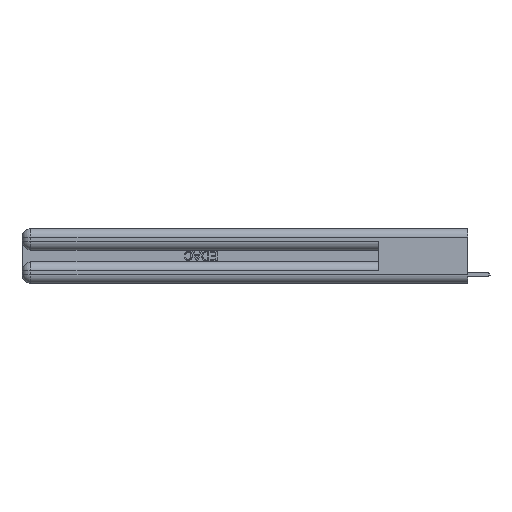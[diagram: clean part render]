
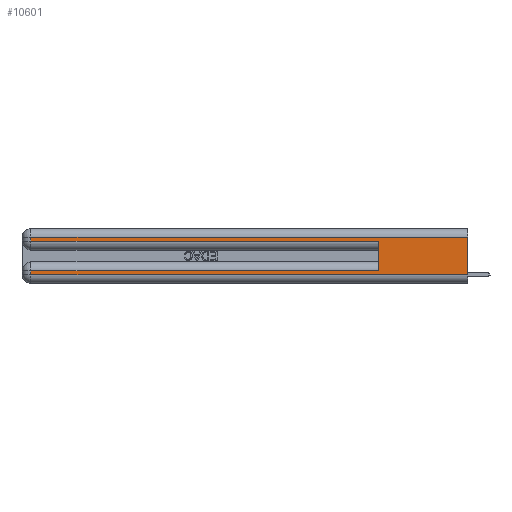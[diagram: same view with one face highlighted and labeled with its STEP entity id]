
A CAD part, left-side view. The second image highlights one B-rep face of the part: STEP entity #10601.
In plain terms, the highlighted planar face has unit normal (-1, 0, 0).
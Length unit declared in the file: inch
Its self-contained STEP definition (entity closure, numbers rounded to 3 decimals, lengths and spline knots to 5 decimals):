
#235 = DIRECTION ( 'NONE',  ( 0., 1., 0. ) ) ;
#849 = VECTOR ( 'NONE', #20794, 39.37008 ) ;
#1959 = VERTEX_POINT ( 'NONE', #27215 ) ;
#2513 = EDGE_CURVE ( 'NONE', #26763, #18658, #7980, .T. ) ;
#3380 = VECTOR ( 'NONE', #11363, 39.37008 ) ;
#3614 = EDGE_CURVE ( 'NONE', #14412, #7182, #16532, .T. ) ;
#3829 = VECTOR ( 'NONE', #19121, 39.37008 ) ;
#3980 = ORIENTED_EDGE ( 'NONE', *, *, #24137, .T. ) ;
#6697 = CARTESIAN_POINT ( 'NONE',  ( 0., 2.94, 0.285 ) ) ;
#7182 = VERTEX_POINT ( 'NONE', #12680 ) ;
#7229 = LINE ( 'NONE', #23382, #849 ) ;
#7321 = CARTESIAN_POINT ( 'NONE',  ( 0., 2.94, 0.37 ) ) ;
#7705 = LINE ( 'NONE', #12514, #15651 ) ;
#7980 = LINE ( 'NONE', #19742, #14417 ) ;
#8640 = ORIENTED_EDGE ( 'NONE', *, *, #27903, .F. ) ;
#8691 = CARTESIAN_POINT ( 'NONE',  ( 0., 0., 0.31 ) ) ;
#8824 = ORIENTED_EDGE ( 'NONE', *, *, #9949, .T. ) ;
#9354 = CARTESIAN_POINT ( 'NONE',  ( 0., 0.6, 0.285 ) ) ;
#9949 = EDGE_CURVE ( 'NONE', #25643, #26763, #21211, .T. ) ;
#9965 = CARTESIAN_POINT ( 'NONE',  ( 0., 2.94, 0.085 ) ) ;
#10220 = CARTESIAN_POINT ( 'NONE',  ( 0., 0., 0.37 ) ) ;
#10309 = LINE ( 'NONE', #19507, #29468 ) ;
#10521 = DIRECTION ( 'NONE',  ( 0., -1., 0. ) ) ;
#10601 = ADVANCED_FACE ( 'NONE', ( #22336 ), #28748, .F. ) ;
#11363 = DIRECTION ( 'NONE',  ( 0., 0., -1. ) ) ;
#12514 = CARTESIAN_POINT ( 'NONE',  ( 0., 0.6, 0.145 ) ) ;
#12680 = CARTESIAN_POINT ( 'NONE',  ( 0., 0., 0.06 ) ) ;
#13570 = VERTEX_POINT ( 'NONE', #9965 ) ;
#14412 = VERTEX_POINT ( 'NONE', #8691 ) ;
#14417 = VECTOR ( 'NONE', #10521, 39.37008 ) ;
#15651 = VECTOR ( 'NONE', #28736, 39.37008 ) ;
#16106 = ORIENTED_EDGE ( 'NONE', *, *, #22147, .T. ) ;
#16199 = EDGE_CURVE ( 'NONE', #13570, #22298, #7229, .T. ) ;
#16532 = LINE ( 'NONE', #10220, #3829 ) ;
#17022 = LINE ( 'NONE', #21890, #26573 ) ;
#17499 = EDGE_CURVE ( 'NONE', #14412, #25643, #27818, .T. ) ;
#17925 = ORIENTED_EDGE ( 'NONE', *, *, #17499, .T. ) ;
#18658 = VERTEX_POINT ( 'NONE', #9354 ) ;
#19046 = ORIENTED_EDGE ( 'NONE', *, *, #16199, .T. ) ;
#19121 = DIRECTION ( 'NONE',  ( 0., 0., -1. ) ) ;
#19507 = CARTESIAN_POINT ( 'NONE',  ( 0., 0., 0.085 ) ) ;
#19614 = DIRECTION ( 'NONE',  ( 0., 0., -1. ) ) ;
#19742 = CARTESIAN_POINT ( 'NONE',  ( 0., 0., 0.285 ) ) ;
#20079 = DIRECTION ( 'NONE',  ( 1., 0., 0. ) ) ;
#20352 = CARTESIAN_POINT ( 'NONE',  ( 0., 2.94, 0.06 ) ) ;
#20794 = DIRECTION ( 'NONE',  ( 0., 0., -1. ) ) ;
#21211 = LINE ( 'NONE', #7321, #3380 ) ;
#21890 = CARTESIAN_POINT ( 'NONE',  ( 0., 0., 0.06 ) ) ;
#22147 = EDGE_CURVE ( 'NONE', #22298, #7182, #17022, .T. ) ;
#22298 = VERTEX_POINT ( 'NONE', #20352 ) ;
#22336 = FACE_OUTER_BOUND ( 'NONE', #29080, .T. ) ;
#23010 = ORIENTED_EDGE ( 'NONE', *, *, #3614, .F. ) ;
#23297 = CARTESIAN_POINT ( 'NONE',  ( 0., 2.94, 0.31 ) ) ;
#23312 = ORIENTED_EDGE ( 'NONE', *, *, #2513, .T. ) ;
#23382 = CARTESIAN_POINT ( 'NONE',  ( 0., 2.94, 0.37 ) ) ;
#23679 = VECTOR ( 'NONE', #235, 39.37008 ) ;
#24137 = EDGE_CURVE ( 'NONE', #1959, #13570, #10309, .T. ) ;
#25643 = VERTEX_POINT ( 'NONE', #23297 ) ;
#26564 = AXIS2_PLACEMENT_3D ( 'NONE', #29179, #20079, #19614 ) ;
#26573 = VECTOR ( 'NONE', #26657, 39.37008 ) ;
#26657 = DIRECTION ( 'NONE',  ( 0., -1., 0. ) ) ;
#26763 = VERTEX_POINT ( 'NONE', #6697 ) ;
#27215 = CARTESIAN_POINT ( 'NONE',  ( 0., 0.6, 0.085 ) ) ;
#27818 = LINE ( 'NONE', #28249, #23679 ) ;
#27903 = EDGE_CURVE ( 'NONE', #1959, #18658, #7705, .T. ) ;
#28249 = CARTESIAN_POINT ( 'NONE',  ( 0., 0., 0.31 ) ) ;
#28736 = DIRECTION ( 'NONE',  ( 0., 0., 1. ) ) ;
#28748 = PLANE ( 'NONE',  #26564 ) ;
#28793 = DIRECTION ( 'NONE',  ( 0., 1., 0. ) ) ;
#29080 = EDGE_LOOP ( 'NONE', ( #23010, #17925, #8824, #23312, #8640, #3980, #19046, #16106 ) ) ;
#29179 = CARTESIAN_POINT ( 'NONE',  ( 0., 0., 0.37 ) ) ;
#29468 = VECTOR ( 'NONE', #28793, 39.37008 ) ;
